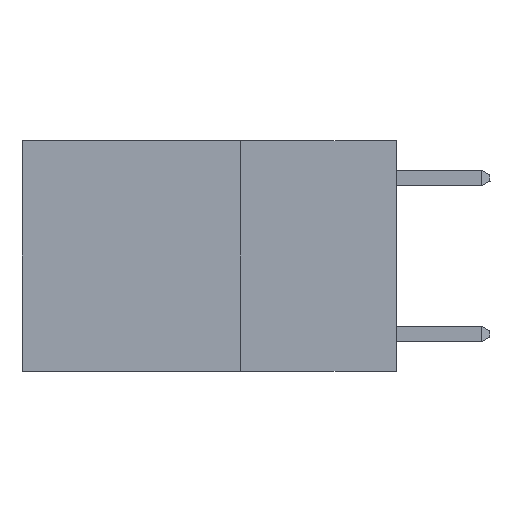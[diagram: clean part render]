
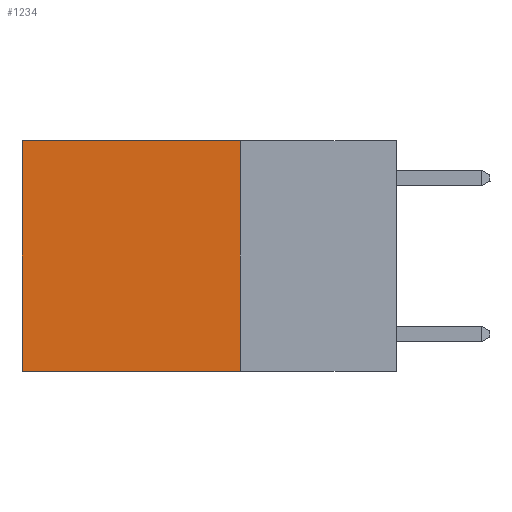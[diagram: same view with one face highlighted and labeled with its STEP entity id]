
A CAD part, left-side view. The second image highlights one B-rep face of the part: STEP entity #1234.
In plain terms, the highlighted planar face has unit normal (-1, 0, 0).
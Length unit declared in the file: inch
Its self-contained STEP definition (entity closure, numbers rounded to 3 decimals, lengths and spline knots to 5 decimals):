
#106 = EDGE_CURVE ( 'NONE', #7230, #4342, #1931, .T. ) ;
#267 = DIRECTION ( 'NONE',  ( 0., 0., -1. ) ) ;
#273 = DIRECTION ( 'NONE',  ( 0., 1., 0. ) ) ;
#593 = VERTEX_POINT ( 'NONE', #3566 ) ;
#812 = EDGE_CURVE ( 'NONE', #593, #2039, #7251, .T. ) ;
#1010 = DIRECTION ( 'NONE',  ( 1., 0., 0. ) ) ;
#1234 = ADVANCED_FACE ( 'NONE', ( #7664 ), #3822, .F. ) ;
#1709 = VECTOR ( 'NONE', #6936, 39.37008 ) ;
#1931 = LINE ( 'NONE', #6143, #3582 ) ;
#1935 = DIRECTION ( 'NONE',  ( 0., 0., -1. ) ) ;
#2039 = VERTEX_POINT ( 'NONE', #8702 ) ;
#2528 = LINE ( 'NONE', #7494, #7606 ) ;
#2787 = ORIENTED_EDGE ( 'NONE', *, *, #7624, .F. ) ;
#3315 = AXIS2_PLACEMENT_3D ( 'NONE', #9113, #1010, #267 ) ;
#3462 = CARTESIAN_POINT ( 'NONE',  ( 0.2625, 0.6, 0. ) ) ;
#3566 = CARTESIAN_POINT ( 'NONE',  ( 0.2625, 0.6, 0. ) ) ;
#3582 = VECTOR ( 'NONE', #1935, 39.37008 ) ;
#3822 = PLANE ( 'NONE',  #3315 ) ;
#4039 = DIRECTION ( 'NONE',  ( 0., 1., 0. ) ) ;
#4342 = VERTEX_POINT ( 'NONE', #7194 ) ;
#5318 = EDGE_CURVE ( 'NONE', #7230, #593, #2528, .T. ) ;
#5411 = CARTESIAN_POINT ( 'NONE',  ( 0.2625, 0.25, -0.37 ) ) ;
#5507 = VECTOR ( 'NONE', #273, 39.37008 ) ;
#5940 = LINE ( 'NONE', #5411, #5507 ) ;
#6143 = CARTESIAN_POINT ( 'NONE',  ( 0.2625, 0.25, 0. ) ) ;
#6266 = ORIENTED_EDGE ( 'NONE', *, *, #5318, .T. ) ;
#6638 = EDGE_LOOP ( 'NONE', ( #8859, #2787, #7246, #6266 ) ) ;
#6936 = DIRECTION ( 'NONE',  ( 0., 0., -1. ) ) ;
#7194 = CARTESIAN_POINT ( 'NONE',  ( 0.2625, 0.25, -0.37 ) ) ;
#7230 = VERTEX_POINT ( 'NONE', #9074 ) ;
#7246 = ORIENTED_EDGE ( 'NONE', *, *, #106, .F. ) ;
#7251 = LINE ( 'NONE', #3462, #1709 ) ;
#7494 = CARTESIAN_POINT ( 'NONE',  ( 0.2625, 0.25, 0. ) ) ;
#7606 = VECTOR ( 'NONE', #4039, 39.37008 ) ;
#7624 = EDGE_CURVE ( 'NONE', #4342, #2039, #5940, .T. ) ;
#7664 = FACE_OUTER_BOUND ( 'NONE', #6638, .T. ) ;
#8702 = CARTESIAN_POINT ( 'NONE',  ( 0.2625, 0.6, -0.37 ) ) ;
#8859 = ORIENTED_EDGE ( 'NONE', *, *, #812, .T. ) ;
#9074 = CARTESIAN_POINT ( 'NONE',  ( 0.2625, 0.25, 0. ) ) ;
#9113 = CARTESIAN_POINT ( 'NONE',  ( 0.2625, 0.25, 0. ) ) ;
